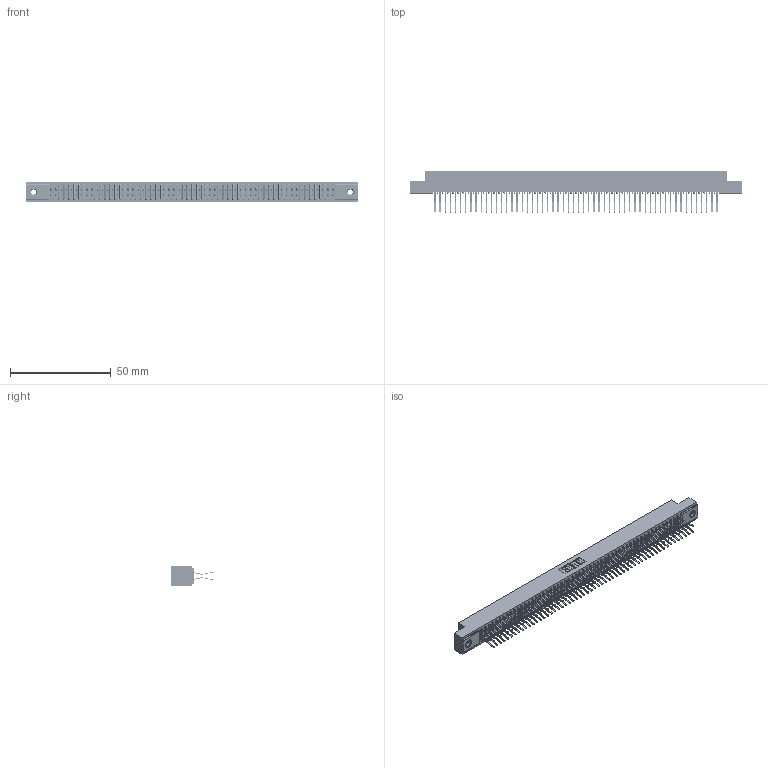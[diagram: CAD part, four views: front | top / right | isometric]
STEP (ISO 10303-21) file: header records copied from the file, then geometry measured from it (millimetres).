
FILE_DESCRIPTION (( 'STEP AP203' ), '1' );
FILE_NAME ('391-112-560-207.STEP', '2018-08-09T22:28:28', ( '' ), ( '' ), 'SwSTEP 2.0', 'SolidWorks 2016', '' );
FILE_SCHEMA (( 'CONFIG_CONTROL_DESIGN' ));
Length unit declared in the file: inch
Products named in the file (4): 391-112-560-207; 341 Part_.156 (3.96) Dia Mounting Holes; 341-292-001_341-292-160; 345-250-001_345-250-005-103
Assembly tree (115 placements, depth 2):
  391-112-560-207
    341 Part_.156 (3.96) Dia Mounting Holes
    341-292-001_341-292-160  x112
    345-250-001_345-250-005-103  x2
Bounding box: 164.47 x 20.37 x 10.16 mm (x, y, z)
Volume: 12255 mm3; surface area: 23060.3 mm2
Topology: 115 solids, 115 shells, 8016 faces, 23244 edges, 15074 vertices
Faces by surface type: plane 4580, cylinder 3196, sphere 114, torus 114, cone 12
Entity records: 67232 total; most frequent: CARTESIAN_POINT 11159, ORIENTED_EDGE 11084, DIRECTION 10834, EDGE_CURVE 5542, VECTOR 4484, LINE 4484, VERTEX_POINT 3500, AXIS2_PLACEMENT_3D 3175
